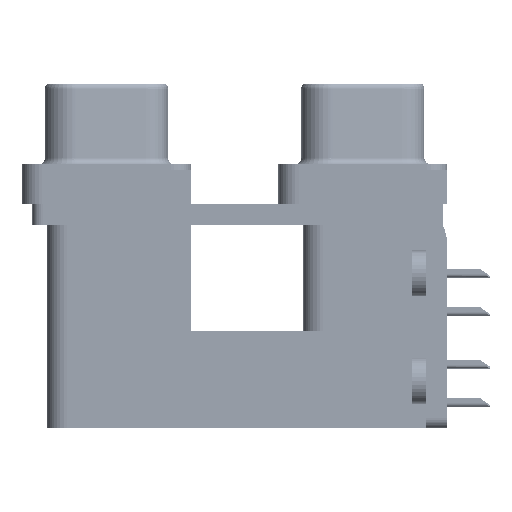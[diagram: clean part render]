
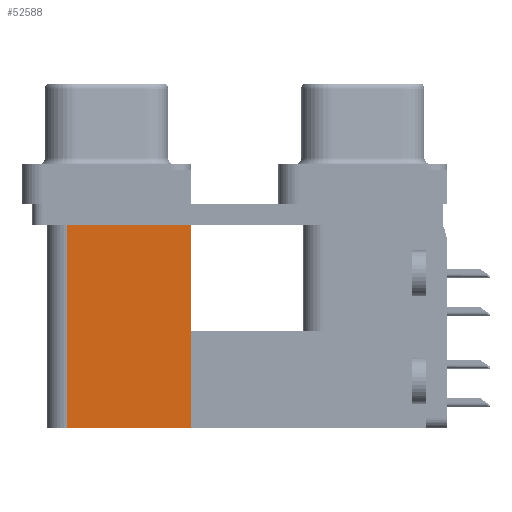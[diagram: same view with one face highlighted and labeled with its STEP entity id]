
A CAD part, left-side view. The second image highlights one B-rep face of the part: STEP entity #52588.
In plain terms, the highlighted planar face has unit normal (-1, 0, 0).
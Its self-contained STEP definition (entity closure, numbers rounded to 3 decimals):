
#619 = FACE_OUTER_BOUND ( 'NONE', #4956, .T. ) ;
#2195 = ORIENTED_EDGE ( 'NONE', *, *, #7522, .F. ) ;
#3173 = CARTESIAN_POINT ( 'NONE',  ( 3.79, 21.975, -2.5 ) ) ;
#4956 = EDGE_LOOP ( 'NONE', ( #51329, #2195, #40192, #15993 ) ) ;
#6931 = VECTOR ( 'NONE', #8005, 1000. ) ;
#7522 = EDGE_CURVE ( 'NONE', #10623, #22559, #49257, .T. ) ;
#8005 = DIRECTION ( 'NONE',  ( 0., 0., 1. ) ) ;
#8307 = CARTESIAN_POINT ( 'NONE',  ( 3.79, 12.775, -19.2 ) ) ;
#10623 = VERTEX_POINT ( 'NONE', #45034 ) ;
#12219 = DIRECTION ( 'NONE',  ( 0., 0., -1. ) ) ;
#13011 = DIRECTION ( 'NONE',  ( 0., 1., 0. ) ) ;
#15993 = ORIENTED_EDGE ( 'NONE', *, *, #43945, .T. ) ;
#17321 = CARTESIAN_POINT ( 'NONE',  ( 3.79, 12.775, -2.5 ) ) ;
#19305 = DIRECTION ( 'NONE',  ( 0., 0., 1. ) ) ;
#19705 = VECTOR ( 'NONE', #19305, 1000. ) ;
#20094 = LINE ( 'NONE', #28176, #19705 ) ;
#20227 = CARTESIAN_POINT ( 'NONE',  ( 3.79, 12.775, -19.2 ) ) ;
#22024 = VECTOR ( 'NONE', #32366, 1000. ) ;
#22078 = AXIS2_PLACEMENT_3D ( 'NONE', #48883, #41078, #12219 ) ;
#22559 = VERTEX_POINT ( 'NONE', #3173 ) ;
#24999 = EDGE_CURVE ( 'NONE', #39064, #10623, #40478, .T. ) ;
#25144 = PLANE ( 'NONE',  #22078 ) ;
#28176 = CARTESIAN_POINT ( 'NONE',  ( 3.79, 12.775, -19.2 ) ) ;
#32366 = DIRECTION ( 'NONE',  ( 0., 1., 0. ) ) ;
#36453 = EDGE_CURVE ( 'NONE', #41715, #22559, #49960, .T. ) ;
#39064 = VERTEX_POINT ( 'NONE', #8307 ) ;
#40192 = ORIENTED_EDGE ( 'NONE', *, *, #24999, .F. ) ;
#40478 = LINE ( 'NONE', #20227, #22024 ) ;
#41078 = DIRECTION ( 'NONE',  ( 1., 0., 0. ) ) ;
#41715 = VERTEX_POINT ( 'NONE', #45628 ) ;
#42530 = VECTOR ( 'NONE', #13011, 1000. ) ;
#43945 = EDGE_CURVE ( 'NONE', #39064, #41715, #20094, .T. ) ;
#45034 = CARTESIAN_POINT ( 'NONE',  ( 3.79, 21.975, -19.2 ) ) ;
#45628 = CARTESIAN_POINT ( 'NONE',  ( 3.79, 12.775, -2.5 ) ) ;
#48883 = CARTESIAN_POINT ( 'NONE',  ( 3.79, 12.775, -19.2 ) ) ;
#49257 = LINE ( 'NONE', #53305, #6931 ) ;
#49960 = LINE ( 'NONE', #17321, #42530 ) ;
#51329 = ORIENTED_EDGE ( 'NONE', *, *, #36453, .T. ) ;
#52588 = ADVANCED_FACE ( 'NONE', ( #619 ), #25144, .F. ) ;
#53305 = CARTESIAN_POINT ( 'NONE',  ( 3.79, 21.975, -19.2 ) ) ;
